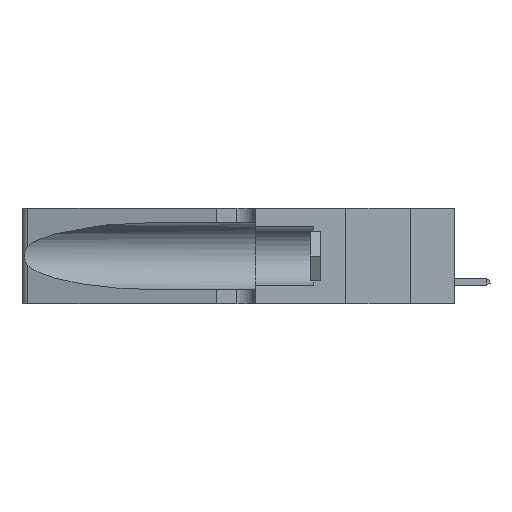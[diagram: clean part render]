
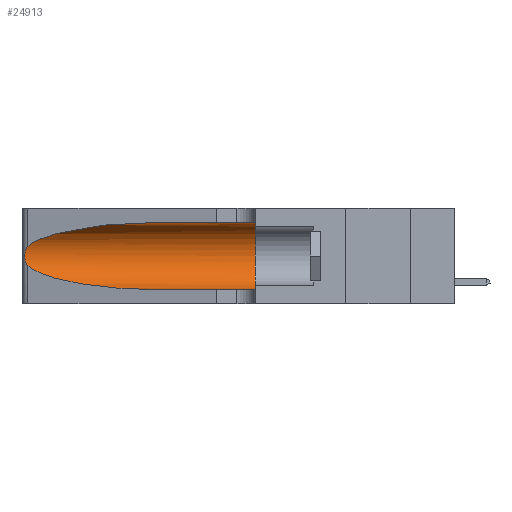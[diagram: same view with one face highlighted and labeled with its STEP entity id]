
A CAD part, left-side view. The second image highlights one B-rep face of the part: STEP entity #24913.
In plain terms, the highlighted cylindrical face has radius 3.308 mm (diameter 6.617 mm), a partial arc.
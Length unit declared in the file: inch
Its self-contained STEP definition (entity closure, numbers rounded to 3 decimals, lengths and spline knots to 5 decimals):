
#29 = VERTEX_POINT ( 'NONE', #17101 ) ;
#402 = LINE ( 'NONE', #15253, #10904 ) ;
#826 = CARTESIAN_POINT ( 'NONE',  ( 0.1305, 0.72297, 0.31525 ) ) ;
#1351 = CARTESIAN_POINT ( 'NONE',  ( 0.25854, 1.2359, 0.20912 ) ) ;
#3510 = CARTESIAN_POINT ( 'NONE',  ( 0.25639, 1.23186, 0.15144 ) ) ;
#3802 = EDGE_CURVE ( 'NONE', #10221, #29, #6103, .T. ) ;
#4565 = ORIENTED_EDGE ( 'NONE', *, *, #3802, .T. ) ;
#4810 = CIRCLE ( 'NONE', #17562, 0.13025 ) ;
#5313 = DIRECTION ( 'NONE',  ( 0., -1., 0. ) ) ;
#5575 = AXIS2_PLACEMENT_3D ( 'NONE', #8202, #10403, #22863 ) ;
#5960 = CARTESIAN_POINT ( 'NONE',  ( 0.1305, 0.72297, 0.05475 ) ) ;
#6103 =( BOUNDED_CURVE ( )  B_SPLINE_CURVE ( 3, ( #26770, #10028, #14195, #18307 ),
 .UNSPECIFIED., .F., .T. ) 
 B_SPLINE_CURVE_WITH_KNOTS ( ( 4, 4 ),
 ( 1.5708, 2.84003 ),
 .UNSPECIFIED. ) 
 CURVE ( )  GEOMETRIC_REPRESENTATION_ITEM ( )  RATIONAL_B_SPLINE_CURVE ( ( 1., 0.87, 0.87, 1. ) ) 
 REPRESENTATION_ITEM ( '' )  );
#6785 = ORIENTED_EDGE ( 'NONE', *, *, #15758, .F. ) ;
#7164 = ORIENTED_EDGE ( 'NONE', *, *, #23580, .T. ) ;
#7814 = CARTESIAN_POINT ( 'NONE',  ( 0.25487, 1.22718, 0.22369 ) ) ;
#7904 = CARTESIAN_POINT ( 'NONE',  ( 0.25555, 1.22993, 0.14849 ) ) ;
#8202 = CARTESIAN_POINT ( 'NONE',  ( 0.1305, 1.61858, 0.185 ) ) ;
#8410 = ORIENTED_EDGE ( 'NONE', *, *, #22119, .T. ) ;
#8824 = LINE ( 'NONE', #20016, #25554 ) ;
#9094 = B_SPLINE_CURVE_WITH_KNOTS ( 'NONE', 3,
 ( #7814, #9845, #12172, #20119, #1351, #22218, #9745, #16085, #9644, #9936, #18381, #3510, #7904, #14189 ),
 .UNSPECIFIED., .F., .F.,
 ( 4, 2, 2, 2, 2, 2, 4 ),
 ( 0., 0.00027, 0.00053, 0.00107, 0.0016, 0.00187, 0.00214 ),
 .UNSPECIFIED. ) ;
#9644 = CARTESIAN_POINT ( 'NONE',  ( 0.26017, 1.23833, 0.17102 ) ) ;
#9745 = CARTESIAN_POINT ( 'NONE',  ( 0.26075, 1.23896, 0.19203 ) ) ;
#9845 = CARTESIAN_POINT ( 'NONE',  ( 0.25555, 1.22994, 0.2215 ) ) ;
#9936 = CARTESIAN_POINT ( 'NONE',  ( 0.25856, 1.23593, 0.16098 ) ) ;
#10028 = CARTESIAN_POINT ( 'NONE',  ( 0.18966, 0.96281, 0.31525 ) ) ;
#10221 = VERTEX_POINT ( 'NONE', #826 ) ;
#10328 = CYLINDRICAL_SURFACE ( 'NONE', #5575, 0.13025 ) ;
#10355 = DIRECTION ( 'NONE',  ( 0., 1., 0. ) ) ;
#10403 = DIRECTION ( 'NONE',  ( 0., -1., 0. ) ) ;
#10904 = VECTOR ( 'NONE', #5313, 39.37008 ) ;
#11539 = EDGE_CURVE ( 'NONE', #10221, #16064, #402, .T. ) ;
#11715 = VERTEX_POINT ( 'NONE', #22555 ) ;
#12172 = CARTESIAN_POINT ( 'NONE',  ( 0.25639, 1.23184, 0.21858 ) ) ;
#12359 =( BOUNDED_CURVE ( )  B_SPLINE_CURVE ( 3, ( #19199, #12891, #21471, #23209 ),
 .UNSPECIFIED., .F., .F. ) 
 B_SPLINE_CURVE_WITH_KNOTS ( ( 4, 4 ),
 ( 3.44316, 4.71239 ),
 .UNSPECIFIED. ) 
 CURVE ( )  GEOMETRIC_REPRESENTATION_ITEM ( )  RATIONAL_B_SPLINE_CURVE ( ( 1., 0.87, 0.87, 1. ) ) 
 REPRESENTATION_ITEM ( '' )  );
#12819 = EDGE_CURVE ( 'NONE', #24482, #26570, #8824, .T. ) ;
#12891 = CARTESIAN_POINT ( 'NONE',  ( 0.2373, 1.15595, 0.08982 ) ) ;
#12972 = FACE_OUTER_BOUND ( 'NONE', #20545, .T. ) ;
#14189 = CARTESIAN_POINT ( 'NONE',  ( 0.25487, 1.22718, 0.14631 ) ) ;
#14195 = CARTESIAN_POINT ( 'NONE',  ( 0.2373, 1.15595, 0.28018 ) ) ;
#15253 = CARTESIAN_POINT ( 'NONE',  ( 0.1305, 1.61858, 0.31525 ) ) ;
#15667 = CARTESIAN_POINT ( 'NONE',  ( 0.1305, 0.35, 0.31525 ) ) ;
#15758 = EDGE_CURVE ( 'NONE', #16064, #26570, #4810, .T. ) ;
#16064 = VERTEX_POINT ( 'NONE', #15667 ) ;
#16085 = CARTESIAN_POINT ( 'NONE',  ( 0.26075, 1.23896, 0.178 ) ) ;
#17101 = CARTESIAN_POINT ( 'NONE',  ( 0.25487, 1.22718, 0.22369 ) ) ;
#17562 = AXIS2_PLACEMENT_3D ( 'NONE', #18708, #10355, #18443 ) ;
#17932 = DIRECTION ( 'NONE',  ( 0., -1., 0. ) ) ;
#18024 = ORIENTED_EDGE ( 'NONE', *, *, #11539, .F. ) ;
#18307 = CARTESIAN_POINT ( 'NONE',  ( 0.25487, 1.22718, 0.22369 ) ) ;
#18381 = CARTESIAN_POINT ( 'NONE',  ( 0.25789, 1.23486, 0.15765 ) ) ;
#18443 = DIRECTION ( 'NONE',  ( 0., 0., 1. ) ) ;
#18708 = CARTESIAN_POINT ( 'NONE',  ( 0.1305, 0.35, 0.185 ) ) ;
#19199 = CARTESIAN_POINT ( 'NONE',  ( 0.25487, 1.22718, 0.14631 ) ) ;
#20016 = CARTESIAN_POINT ( 'NONE',  ( 0.1305, 1.61858, 0.05475 ) ) ;
#20119 = CARTESIAN_POINT ( 'NONE',  ( 0.25787, 1.23484, 0.2124 ) ) ;
#20545 = EDGE_LOOP ( 'NONE', ( #4565, #7164, #8410, #22464, #6785, #18024 ) ) ;
#21471 = CARTESIAN_POINT ( 'NONE',  ( 0.18966, 0.96281, 0.05475 ) ) ;
#22119 = EDGE_CURVE ( 'NONE', #11715, #24482, #12359, .T. ) ;
#22218 = CARTESIAN_POINT ( 'NONE',  ( 0.26018, 1.23835, 0.19895 ) ) ;
#22464 = ORIENTED_EDGE ( 'NONE', *, *, #12819, .T. ) ;
#22555 = CARTESIAN_POINT ( 'NONE',  ( 0.25487, 1.22718, 0.14631 ) ) ;
#22863 = DIRECTION ( 'NONE',  ( 0., 0., -1. ) ) ;
#23209 = CARTESIAN_POINT ( 'NONE',  ( 0.1305, 0.72297, 0.05475 ) ) ;
#23580 = EDGE_CURVE ( 'NONE', #29, #11715, #9094, .T. ) ;
#24482 = VERTEX_POINT ( 'NONE', #5960 ) ;
#24913 = ADVANCED_FACE ( 'NONE', ( #12972 ), #10328, .F. ) ;
#25506 = CARTESIAN_POINT ( 'NONE',  ( 0.1305, 0.35, 0.05475 ) ) ;
#25554 = VECTOR ( 'NONE', #17932, 39.37008 ) ;
#26570 = VERTEX_POINT ( 'NONE', #25506 ) ;
#26770 = CARTESIAN_POINT ( 'NONE',  ( 0.1305, 0.72297, 0.31525 ) ) ;
